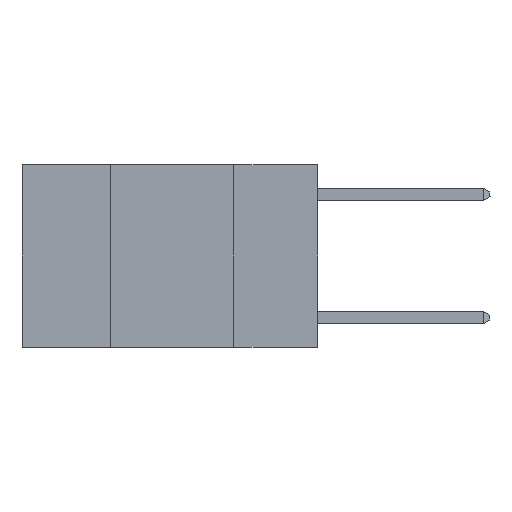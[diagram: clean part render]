
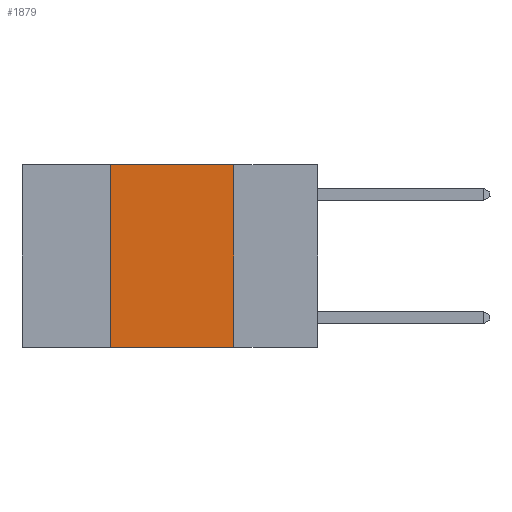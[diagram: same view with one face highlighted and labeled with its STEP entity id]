
A CAD part, left-side view. The second image highlights one B-rep face of the part: STEP entity #1879.
In plain terms, the highlighted planar face has unit normal (-1, 0, 0).
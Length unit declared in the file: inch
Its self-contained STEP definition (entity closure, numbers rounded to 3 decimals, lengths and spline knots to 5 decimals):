
#46 = EDGE_CURVE ( 'NONE', #5458, #1183, #10399, .T. ) ;
#116 = VERTEX_POINT ( 'NONE', #9877 ) ;
#1002 = DIRECTION ( 'NONE',  ( 0., 0., -1. ) ) ;
#1158 = VERTEX_POINT ( 'NONE', #12827 ) ;
#1183 = VERTEX_POINT ( 'NONE', #6946 ) ;
#1879 = ADVANCED_FACE ( 'NONE', ( #13152 ), #4302, .F. ) ;
#1900 = LINE ( 'NONE', #13583, #10138 ) ;
#2208 = CARTESIAN_POINT ( 'NONE',  ( 0., 0.42, 0. ) ) ;
#2815 = CARTESIAN_POINT ( 'NONE',  ( 0., 0.42, 0. ) ) ;
#2931 = DIRECTION ( 'NONE',  ( 0., -1., 0. ) ) ;
#3600 = EDGE_CURVE ( 'NONE', #1158, #5458, #12326, .T. ) ;
#4302 = PLANE ( 'NONE',  #5805 ) ;
#5190 = CARTESIAN_POINT ( 'NONE',  ( 0., 0.6, -0.37 ) ) ;
#5398 = DIRECTION ( 'NONE',  ( 0., 0., -1. ) ) ;
#5458 = VERTEX_POINT ( 'NONE', #2208 ) ;
#5805 = AXIS2_PLACEMENT_3D ( 'NONE', #12686, #11728, #5398 ) ;
#6352 = DIRECTION ( 'NONE',  ( 0., -1., 0. ) ) ;
#6946 = CARTESIAN_POINT ( 'NONE',  ( 0., 0.17, 0. ) ) ;
#7744 = EDGE_CURVE ( 'NONE', #1183, #116, #1900, .T. ) ;
#8212 = DIRECTION ( 'NONE',  ( 0., 0., 1. ) ) ;
#9877 = CARTESIAN_POINT ( 'NONE',  ( 0., 0.17, -0.37 ) ) ;
#10097 = ORIENTED_EDGE ( 'NONE', *, *, #46, .F. ) ;
#10138 = VECTOR ( 'NONE', #1002, 39.37008 ) ;
#10211 = VECTOR ( 'NONE', #6352, 39.37008 ) ;
#10375 = EDGE_LOOP ( 'NONE', ( #12118, #10097, #10415, #13079 ) ) ;
#10399 = LINE ( 'NONE', #10959, #12755 ) ;
#10415 = ORIENTED_EDGE ( 'NONE', *, *, #3600, .F. ) ;
#10959 = CARTESIAN_POINT ( 'NONE',  ( 0., 0.6, 0. ) ) ;
#11035 = EDGE_CURVE ( 'NONE', #1158, #116, #12889, .T. ) ;
#11728 = DIRECTION ( 'NONE',  ( 1., 0., 0. ) ) ;
#12013 = VECTOR ( 'NONE', #8212, 39.37008 ) ;
#12118 = ORIENTED_EDGE ( 'NONE', *, *, #7744, .F. ) ;
#12326 = LINE ( 'NONE', #2815, #12013 ) ;
#12686 = CARTESIAN_POINT ( 'NONE',  ( 0., 0.6, 0. ) ) ;
#12755 = VECTOR ( 'NONE', #2931, 39.37008 ) ;
#12827 = CARTESIAN_POINT ( 'NONE',  ( 0., 0.42, -0.37 ) ) ;
#12889 = LINE ( 'NONE', #5190, #10211 ) ;
#13079 = ORIENTED_EDGE ( 'NONE', *, *, #11035, .T. ) ;
#13152 = FACE_OUTER_BOUND ( 'NONE', #10375, .T. ) ;
#13583 = CARTESIAN_POINT ( 'NONE',  ( 0., 0.17, 0. ) ) ;
